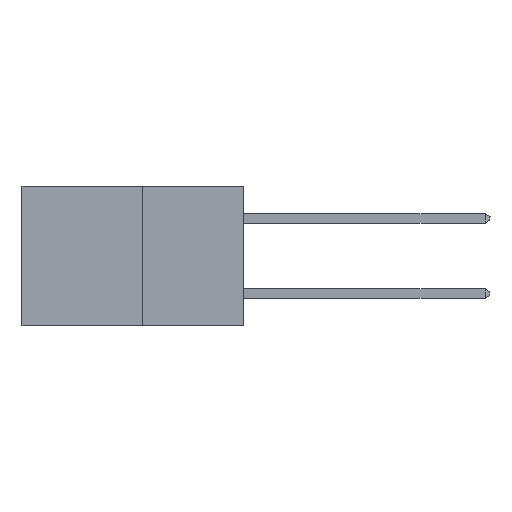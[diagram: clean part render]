
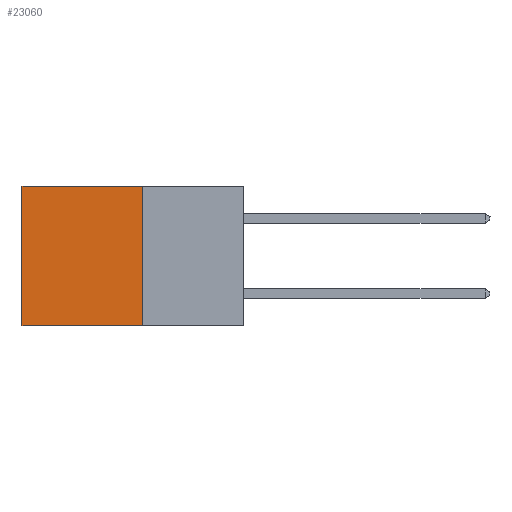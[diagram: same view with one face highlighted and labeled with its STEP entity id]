
A CAD part, left-side view. The second image highlights one B-rep face of the part: STEP entity #23060.
In plain terms, the highlighted planar face has unit normal (-1, 0, 0).
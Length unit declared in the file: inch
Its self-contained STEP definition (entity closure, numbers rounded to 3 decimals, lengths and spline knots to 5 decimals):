
#15 = DIRECTION ( 'NONE',  ( 0., 0., -1. ) ) ;
#1239 = DIRECTION ( 'NONE',  ( 1., 0., 0. ) ) ;
#1300 = FACE_OUTER_BOUND ( 'NONE', #7552, .T. ) ;
#2060 = CARTESIAN_POINT ( 'NONE',  ( 0.277, 0.59, -0.37 ) ) ;
#3500 = ORIENTED_EDGE ( 'NONE', *, *, #8050, .T. ) ;
#3914 = ORIENTED_EDGE ( 'NONE', *, *, #12009, .F. ) ;
#4189 = EDGE_CURVE ( 'NONE', #17256, #15797, #9675, .T. ) ;
#4397 = AXIS2_PLACEMENT_3D ( 'NONE', #25271, #1239, #15416 ) ;
#4460 = VERTEX_POINT ( 'NONE', #2060 ) ;
#7552 = EDGE_LOOP ( 'NONE', ( #3500, #23459, #3914, #19101 ) ) ;
#7917 = CARTESIAN_POINT ( 'NONE',  ( 0.277, 0.27, 0. ) ) ;
#8050 = EDGE_CURVE ( 'NONE', #15797, #4460, #25145, .T. ) ;
#8236 = DIRECTION ( 'NONE',  ( 0., 1., 0. ) ) ;
#8617 = CARTESIAN_POINT ( 'NONE',  ( 0.277, 0.27, 0. ) ) ;
#8916 = EDGE_CURVE ( 'NONE', #24967, #4460, #15545, .T. ) ;
#9039 = VECTOR ( 'NONE', #8236, 39.37008 ) ;
#9675 = LINE ( 'NONE', #8617, #9039 ) ;
#10178 = CARTESIAN_POINT ( 'NONE',  ( 0.277, 0.27, -0.37 ) ) ;
#11723 = CARTESIAN_POINT ( 'NONE',  ( 0.277, 0.59, 0. ) ) ;
#12009 = EDGE_CURVE ( 'NONE', #17256, #24967, #13162, .T. ) ;
#13162 = LINE ( 'NONE', #10178, #17841 ) ;
#13413 = PLANE ( 'NONE',  #4397 ) ;
#14531 = VECTOR ( 'NONE', #18679, 39.37008 ) ;
#14757 = CARTESIAN_POINT ( 'NONE',  ( 0.277, 0.59, -0.37 ) ) ;
#15416 = DIRECTION ( 'NONE',  ( 0., 0., -1. ) ) ;
#15545 = LINE ( 'NONE', #17679, #19597 ) ;
#15760 = DIRECTION ( 'NONE',  ( 0., 1., 0. ) ) ;
#15797 = VERTEX_POINT ( 'NONE', #11723 ) ;
#17256 = VERTEX_POINT ( 'NONE', #7917 ) ;
#17679 = CARTESIAN_POINT ( 'NONE',  ( 0.277, 0.27, -0.37 ) ) ;
#17841 = VECTOR ( 'NONE', #15, 39.37008 ) ;
#18679 = DIRECTION ( 'NONE',  ( 0., 0., -1. ) ) ;
#19101 = ORIENTED_EDGE ( 'NONE', *, *, #4189, .T. ) ;
#19597 = VECTOR ( 'NONE', #15760, 39.37008 ) ;
#22091 = CARTESIAN_POINT ( 'NONE',  ( 0.277, 0.27, -0.37 ) ) ;
#23060 = ADVANCED_FACE ( 'NONE', ( #1300 ), #13413, .F. ) ;
#23459 = ORIENTED_EDGE ( 'NONE', *, *, #8916, .F. ) ;
#24967 = VERTEX_POINT ( 'NONE', #22091 ) ;
#25145 = LINE ( 'NONE', #14757, #14531 ) ;
#25271 = CARTESIAN_POINT ( 'NONE',  ( 0.277, 0.27, -0.37 ) ) ;
